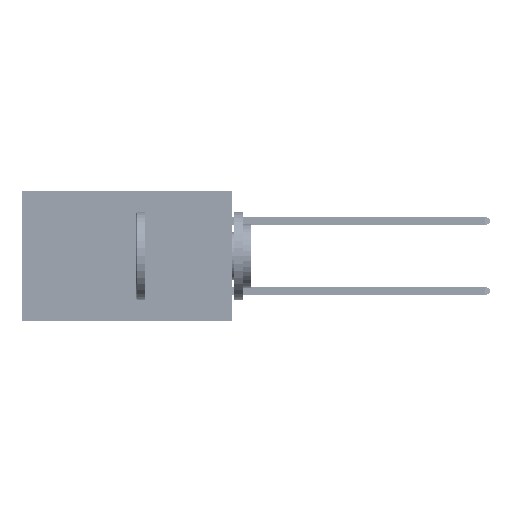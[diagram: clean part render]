
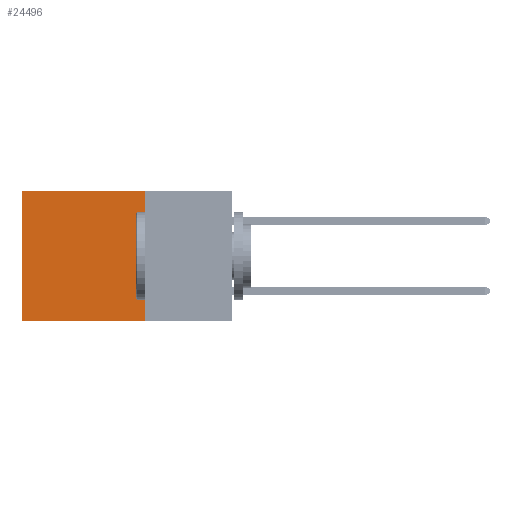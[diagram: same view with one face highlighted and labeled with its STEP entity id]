
A CAD part, left-side view. The second image highlights one B-rep face of the part: STEP entity #24496.
In plain terms, the highlighted planar face has unit normal (-1, 0, 0).
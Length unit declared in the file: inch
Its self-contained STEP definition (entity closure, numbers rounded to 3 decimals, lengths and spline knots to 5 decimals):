
#2342 = CARTESIAN_POINT ( 'NONE',  ( 0.2875, 0.25, -0.37 ) ) ;
#4062 = VECTOR ( 'NONE', #8199, 39.37008 ) ;
#4746 = EDGE_LOOP ( 'NONE', ( #10895, #32706, #5959, #42836 ) ) ;
#5959 = ORIENTED_EDGE ( 'NONE', *, *, #16752, .F. ) ;
#6940 = EDGE_CURVE ( 'NONE', #11389, #13517, #17978, .T. ) ;
#7897 = DIRECTION ( 'NONE',  ( 0., 1., 0. ) ) ;
#8199 = DIRECTION ( 'NONE',  ( 0., 1., 0. ) ) ;
#10895 = ORIENTED_EDGE ( 'NONE', *, *, #6940, .T. ) ;
#11389 = VERTEX_POINT ( 'NONE', #15962 ) ;
#12116 = EDGE_CURVE ( 'NONE', #34780, #11389, #41791, .T. ) ;
#13517 = VERTEX_POINT ( 'NONE', #37999 ) ;
#15134 = LINE ( 'NONE', #20459, #4062 ) ;
#15593 = CARTESIAN_POINT ( 'NONE',  ( 0.2875, 0.6, 0. ) ) ;
#15962 = CARTESIAN_POINT ( 'NONE',  ( 0.2875, 0.6, 0. ) ) ;
#16752 = EDGE_CURVE ( 'NONE', #34780, #29534, #39258, .T. ) ;
#17978 = LINE ( 'NONE', #15593, #49256 ) ;
#18828 = CARTESIAN_POINT ( 'NONE',  ( 0.2875, 0.25, 0. ) ) ;
#20459 = CARTESIAN_POINT ( 'NONE',  ( 0.2875, 0.25, -0.37 ) ) ;
#24496 = ADVANCED_FACE ( 'NONE', ( #24881 ), #43293, .F. ) ;
#24881 = FACE_OUTER_BOUND ( 'NONE', #4746, .T. ) ;
#27048 = DIRECTION ( 'NONE',  ( 0., 0., -1. ) ) ;
#27971 = DIRECTION ( 'NONE',  ( 0., 0., -1. ) ) ;
#29534 = VERTEX_POINT ( 'NONE', #2342 ) ;
#30930 = VECTOR ( 'NONE', #7897, 39.37008 ) ;
#32511 = CARTESIAN_POINT ( 'NONE',  ( 0.2875, 0.25, 0. ) ) ;
#32706 = ORIENTED_EDGE ( 'NONE', *, *, #44281, .F. ) ;
#34780 = VERTEX_POINT ( 'NONE', #48710 ) ;
#35976 = DIRECTION ( 'NONE',  ( 0., 0., -1. ) ) ;
#37951 = VECTOR ( 'NONE', #27971, 39.37008 ) ;
#37999 = CARTESIAN_POINT ( 'NONE',  ( 0.2875, 0.6, -0.37 ) ) ;
#39258 = LINE ( 'NONE', #44209, #37951 ) ;
#41791 = LINE ( 'NONE', #32511, #30930 ) ;
#42836 = ORIENTED_EDGE ( 'NONE', *, *, #12116, .T. ) ;
#43293 = PLANE ( 'NONE',  #48791 ) ;
#44209 = CARTESIAN_POINT ( 'NONE',  ( 0.2875, 0.25, 0. ) ) ;
#44281 = EDGE_CURVE ( 'NONE', #29534, #13517, #15134, .T. ) ;
#48710 = CARTESIAN_POINT ( 'NONE',  ( 0.2875, 0.25, 0. ) ) ;
#48791 = AXIS2_PLACEMENT_3D ( 'NONE', #18828, #51478, #27048 ) ;
#49256 = VECTOR ( 'NONE', #35976, 39.37008 ) ;
#51478 = DIRECTION ( 'NONE',  ( 1., 0., 0. ) ) ;
